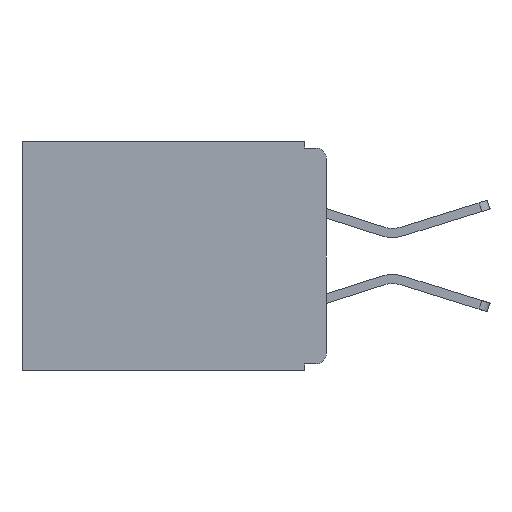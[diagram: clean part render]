
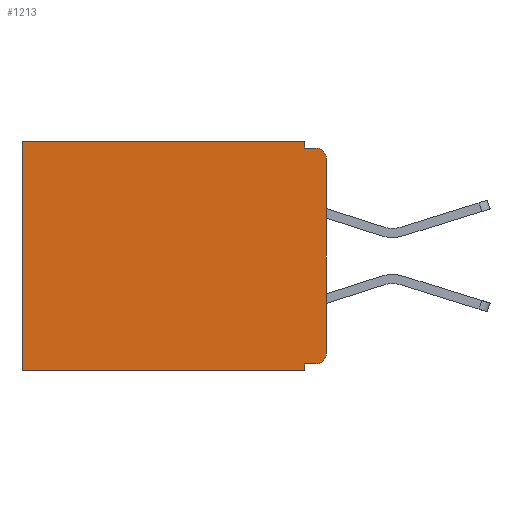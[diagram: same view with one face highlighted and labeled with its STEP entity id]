
A CAD part, left-side view. The second image highlights one B-rep face of the part: STEP entity #1213.
In plain terms, the highlighted planar face has unit normal (-1, 0, 0).
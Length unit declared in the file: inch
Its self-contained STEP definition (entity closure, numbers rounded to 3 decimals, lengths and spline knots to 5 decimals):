
#4 = ORIENTED_EDGE ( 'NONE', *, *, #10598, .F. ) ;
#87 = VECTOR ( 'NONE', #5998, 39.37008 ) ;
#192 = CIRCLE ( 'NONE', #12303, 0.015 ) ;
#613 = EDGE_CURVE ( 'NONE', #1561, #7695, #8361, .T. ) ;
#719 = CARTESIAN_POINT ( 'NONE',  ( 0.3, 0.031, -0.33 ) ) ;
#736 = FACE_OUTER_BOUND ( 'NONE', #12254, .T. ) ;
#840 = VERTEX_POINT ( 'NONE', #719 ) ;
#860 = EDGE_CURVE ( 'NONE', #5516, #6204, #8856, .T. ) ;
#864 = CARTESIAN_POINT ( 'NONE',  ( 0.3, 0.437, -0.33 ) ) ;
#1192 = CARTESIAN_POINT ( 'NONE',  ( 0.3, 0.015, -0.025 ) ) ;
#1213 = ADVANCED_FACE ( 'NONE', ( #736 ), #12556, .F. ) ;
#1252 = DIRECTION ( 'NONE',  ( 0., 1., 0. ) ) ;
#1283 = DIRECTION ( 'NONE',  ( 0., 0., -1. ) ) ;
#1397 = EDGE_CURVE ( 'NONE', #13518, #13620, #1950, .T. ) ;
#1533 = ORIENTED_EDGE ( 'NONE', *, *, #7660, .F. ) ;
#1561 = VERTEX_POINT ( 'NONE', #8772 ) ;
#1646 = CARTESIAN_POINT ( 'NONE',  ( 0.3, 0., 0. ) ) ;
#1950 = LINE ( 'NONE', #13231, #4230 ) ;
#1960 = VECTOR ( 'NONE', #1252, 39.37008 ) ;
#2004 = CARTESIAN_POINT ( 'NONE',  ( 0.3, 0., -0.01 ) ) ;
#2063 = LINE ( 'NONE', #5191, #12643 ) ;
#2632 = CARTESIAN_POINT ( 'NONE',  ( 0.3, 0., -0.32 ) ) ;
#2945 = ORIENTED_EDGE ( 'NONE', *, *, #9540, .F. ) ;
#3145 = DIRECTION ( 'NONE',  ( 0., -1., 0. ) ) ;
#3193 = CARTESIAN_POINT ( 'NONE',  ( 0.3, 0.031, -0.01 ) ) ;
#3353 = CARTESIAN_POINT ( 'NONE',  ( 0.3, 0.015, -0.305 ) ) ;
#3678 = AXIS2_PLACEMENT_3D ( 'NONE', #3353, #10032, #1283 ) ;
#3944 = EDGE_CURVE ( 'NONE', #5516, #10550, #4527, .T. ) ;
#4230 = VECTOR ( 'NONE', #13951, 39.37008 ) ;
#4527 = CIRCLE ( 'NONE', #3678, 0.015 ) ;
#4543 = DIRECTION ( 'NONE',  ( -1., 0., 0. ) ) ;
#4887 = ORIENTED_EDGE ( 'NONE', *, *, #860, .F. ) ;
#5191 = CARTESIAN_POINT ( 'NONE',  ( 0.3, 0., -0.33 ) ) ;
#5235 = ORIENTED_EDGE ( 'NONE', *, *, #10107, .F. ) ;
#5465 = VECTOR ( 'NONE', #6904, 39.37008 ) ;
#5516 = VERTEX_POINT ( 'NONE', #11340 ) ;
#5998 = DIRECTION ( 'NONE',  ( 0., 1., 0. ) ) ;
#6182 = CARTESIAN_POINT ( 'NONE',  ( 0.3, 0.031, -0.32 ) ) ;
#6204 = VERTEX_POINT ( 'NONE', #6182 ) ;
#6904 = DIRECTION ( 'NONE',  ( 0., 0., -1. ) ) ;
#7004 = VECTOR ( 'NONE', #8251, 39.37008 ) ;
#7069 = CARTESIAN_POINT ( 'NONE',  ( 0.3, 0.015, -0.01 ) ) ;
#7080 = EDGE_CURVE ( 'NONE', #13278, #13083, #192, .T. ) ;
#7471 = ORIENTED_EDGE ( 'NONE', *, *, #3944, .T. ) ;
#7579 = DIRECTION ( 'NONE',  ( 0., 0., -1. ) ) ;
#7600 = ORIENTED_EDGE ( 'NONE', *, *, #10499, .T. ) ;
#7660 = EDGE_CURVE ( 'NONE', #13278, #10550, #2063, .T. ) ;
#7695 = VERTEX_POINT ( 'NONE', #3193 ) ;
#7719 = LINE ( 'NONE', #2004, #13740 ) ;
#8251 = DIRECTION ( 'NONE',  ( 0., 1., 0. ) ) ;
#8361 = LINE ( 'NONE', #11662, #5465 ) ;
#8772 = CARTESIAN_POINT ( 'NONE',  ( 0.3, 0.031, 0. ) ) ;
#8856 = LINE ( 'NONE', #2632, #1960 ) ;
#8882 = VECTOR ( 'NONE', #10670, 39.37008 ) ;
#9203 = LINE ( 'NONE', #9570, #8882 ) ;
#9540 = EDGE_CURVE ( 'NONE', #7695, #13083, #7719, .T. ) ;
#9570 = CARTESIAN_POINT ( 'NONE',  ( 0.3, 0.031, -0.33 ) ) ;
#9622 = ORIENTED_EDGE ( 'NONE', *, *, #1397, .T. ) ;
#9878 = LINE ( 'NONE', #1646, #7004 ) ;
#10032 = DIRECTION ( 'NONE',  ( -1., 0., 0. ) ) ;
#10107 = EDGE_CURVE ( 'NONE', #6204, #840, #9203, .T. ) ;
#10499 = EDGE_CURVE ( 'NONE', #1561, #13518, #9878, .T. ) ;
#10543 = DIRECTION ( 'NONE',  ( 0., 0., -1. ) ) ;
#10550 = VERTEX_POINT ( 'NONE', #11308 ) ;
#10598 = EDGE_CURVE ( 'NONE', #840, #13620, #11412, .T. ) ;
#10670 = DIRECTION ( 'NONE',  ( 0., 0., -1. ) ) ;
#10803 = AXIS2_PLACEMENT_3D ( 'NONE', #11036, #11584, #13784 ) ;
#10994 = ORIENTED_EDGE ( 'NONE', *, *, #613, .F. ) ;
#11036 = CARTESIAN_POINT ( 'NONE',  ( 0.3, 0., -0.33 ) ) ;
#11308 = CARTESIAN_POINT ( 'NONE',  ( 0.3, 0., -0.305 ) ) ;
#11340 = CARTESIAN_POINT ( 'NONE',  ( 0.3, 0.015, -0.32 ) ) ;
#11412 = LINE ( 'NONE', #12443, #87 ) ;
#11584 = DIRECTION ( 'NONE',  ( 1., 0., 0. ) ) ;
#11606 = CARTESIAN_POINT ( 'NONE',  ( 0.3, 0.437, 0. ) ) ;
#11662 = CARTESIAN_POINT ( 'NONE',  ( 0.3, 0.031, 0. ) ) ;
#11740 = CARTESIAN_POINT ( 'NONE',  ( 0.3, 0., -0.025 ) ) ;
#12254 = EDGE_LOOP ( 'NONE', ( #1533, #12626, #2945, #10994, #7600, #9622, #4, #5235, #4887, #7471 ) ) ;
#12303 = AXIS2_PLACEMENT_3D ( 'NONE', #1192, #4543, #10543 ) ;
#12443 = CARTESIAN_POINT ( 'NONE',  ( 0.3, 0., -0.33 ) ) ;
#12556 = PLANE ( 'NONE',  #10803 ) ;
#12626 = ORIENTED_EDGE ( 'NONE', *, *, #7080, .T. ) ;
#12643 = VECTOR ( 'NONE', #7579, 39.37008 ) ;
#13083 = VERTEX_POINT ( 'NONE', #7069 ) ;
#13231 = CARTESIAN_POINT ( 'NONE',  ( 0.3, 0.437, -0.33 ) ) ;
#13278 = VERTEX_POINT ( 'NONE', #11740 ) ;
#13518 = VERTEX_POINT ( 'NONE', #11606 ) ;
#13620 = VERTEX_POINT ( 'NONE', #864 ) ;
#13740 = VECTOR ( 'NONE', #3145, 39.37008 ) ;
#13784 = DIRECTION ( 'NONE',  ( 0., 0., -1. ) ) ;
#13951 = DIRECTION ( 'NONE',  ( 0., 0., -1. ) ) ;
